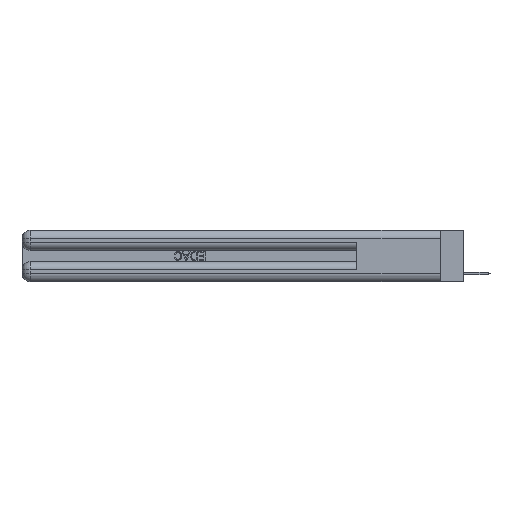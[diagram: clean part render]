
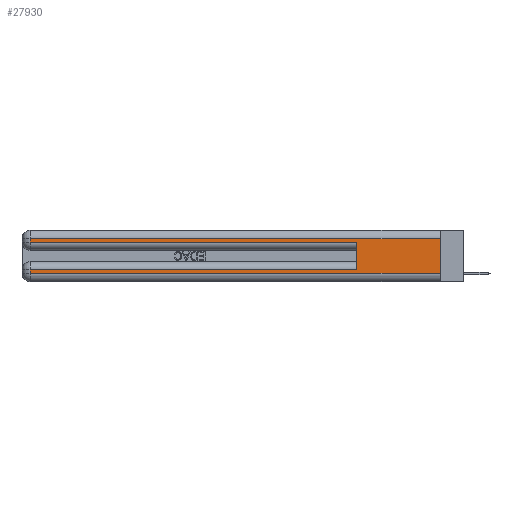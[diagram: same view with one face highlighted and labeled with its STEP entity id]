
A CAD part, left-side view. The second image highlights one B-rep face of the part: STEP entity #27930.
In plain terms, the highlighted planar face has unit normal (-1, 0, 0).
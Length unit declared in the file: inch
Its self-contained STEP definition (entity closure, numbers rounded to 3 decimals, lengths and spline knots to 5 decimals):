
#1215 = ORIENTED_EDGE ( 'NONE', *, *, #13368, .F. ) ;
#2618 = LINE ( 'NONE', #22978, #9329 ) ;
#2910 = CARTESIAN_POINT ( 'NONE',  ( 0., 2.94, 0.37 ) ) ;
#3831 = VECTOR ( 'NONE', #19390, 39.37008 ) ;
#4505 = DIRECTION ( 'NONE',  ( 0., 0., 1. ) ) ;
#5146 = CARTESIAN_POINT ( 'NONE',  ( 0., 2.94, 0.06 ) ) ;
#5337 = EDGE_CURVE ( 'NONE', #7466, #20631, #20648, .T. ) ;
#5552 = ORIENTED_EDGE ( 'NONE', *, *, #7578, .T. ) ;
#6166 = VERTEX_POINT ( 'NONE', #7833 ) ;
#6330 = FACE_OUTER_BOUND ( 'NONE', #6844, .T. ) ;
#6465 = CARTESIAN_POINT ( 'NONE',  ( 0., 0.6, 0.085 ) ) ;
#6713 = ORIENTED_EDGE ( 'NONE', *, *, #5337, .T. ) ;
#6844 = EDGE_LOOP ( 'NONE', ( #1215, #6713, #9039, #5552, #26929, #23325, #10239, #13207 ) ) ;
#7064 = DIRECTION ( 'NONE',  ( 0., 1., 0. ) ) ;
#7466 = VERTEX_POINT ( 'NONE', #10834 ) ;
#7518 = VECTOR ( 'NONE', #18152, 39.37008 ) ;
#7578 = EDGE_CURVE ( 'NONE', #30555, #27766, #29322, .T. ) ;
#7833 = CARTESIAN_POINT ( 'NONE',  ( 0., 2.94, 0.085 ) ) ;
#7868 = LINE ( 'NONE', #21384, #28889 ) ;
#7898 = CARTESIAN_POINT ( 'NONE',  ( 0., 2.94, 0.31 ) ) ;
#8642 = DIRECTION ( 'NONE',  ( 0., 1., 0. ) ) ;
#9039 = ORIENTED_EDGE ( 'NONE', *, *, #16519, .T. ) ;
#9329 = VECTOR ( 'NONE', #7064, 39.37008 ) ;
#9501 = CARTESIAN_POINT ( 'NONE',  ( 0., 2.94, 0.37 ) ) ;
#10239 = ORIENTED_EDGE ( 'NONE', *, *, #20258, .T. ) ;
#10388 = DIRECTION ( 'NONE',  ( 0., 0., -1. ) ) ;
#10834 = CARTESIAN_POINT ( 'NONE',  ( 0., 0., 0.31 ) ) ;
#11643 = DIRECTION ( 'NONE',  ( 0., 0., -1. ) ) ;
#12495 = VECTOR ( 'NONE', #18822, 39.37008 ) ;
#12959 = EDGE_CURVE ( 'NONE', #17915, #25589, #19751, .T. ) ;
#13207 = ORIENTED_EDGE ( 'NONE', *, *, #12959, .T. ) ;
#13304 = VECTOR ( 'NONE', #8642, 39.37008 ) ;
#13368 = EDGE_CURVE ( 'NONE', #7466, #25589, #7868, .T. ) ;
#13879 = VECTOR ( 'NONE', #11643, 39.37008 ) ;
#14038 = CARTESIAN_POINT ( 'NONE',  ( 0., 0.6, 0.285 ) ) ;
#14479 = EDGE_CURVE ( 'NONE', #26904, #6166, #2618, .T. ) ;
#15203 = LINE ( 'NONE', #16037, #24009 ) ;
#15687 = CARTESIAN_POINT ( 'NONE',  ( 0., 0., 0.06 ) ) ;
#15903 = CARTESIAN_POINT ( 'NONE',  ( 0., 2.94, 0.285 ) ) ;
#16037 = CARTESIAN_POINT ( 'NONE',  ( 0., 0.6, 0.145 ) ) ;
#16519 = EDGE_CURVE ( 'NONE', #20631, #30555, #24879, .T. ) ;
#16583 = DIRECTION ( 'NONE',  ( 0., 0., -1. ) ) ;
#17915 = VERTEX_POINT ( 'NONE', #5146 ) ;
#18152 = DIRECTION ( 'NONE',  ( 0., -1., 0. ) ) ;
#18822 = DIRECTION ( 'NONE',  ( 0., 0., -1. ) ) ;
#19390 = DIRECTION ( 'NONE',  ( 0., -1., 0. ) ) ;
#19583 = PLANE ( 'NONE',  #29483 ) ;
#19751 = LINE ( 'NONE', #15687, #7518 ) ;
#20258 = EDGE_CURVE ( 'NONE', #6166, #17915, #23531, .T. ) ;
#20631 = VERTEX_POINT ( 'NONE', #7898 ) ;
#20648 = LINE ( 'NONE', #25354, #13304 ) ;
#21384 = CARTESIAN_POINT ( 'NONE',  ( 0., 0., 0.37 ) ) ;
#22978 = CARTESIAN_POINT ( 'NONE',  ( 0., 0., 0.085 ) ) ;
#22984 = CARTESIAN_POINT ( 'NONE',  ( 0., 0., 0.06 ) ) ;
#23325 = ORIENTED_EDGE ( 'NONE', *, *, #14479, .T. ) ;
#23531 = LINE ( 'NONE', #9501, #12495 ) ;
#23765 = CARTESIAN_POINT ( 'NONE',  ( 0., 0., 0.285 ) ) ;
#24009 = VECTOR ( 'NONE', #4505, 39.37008 ) ;
#24574 = CARTESIAN_POINT ( 'NONE',  ( 0., 0., 0.37 ) ) ;
#24879 = LINE ( 'NONE', #2910, #13879 ) ;
#25354 = CARTESIAN_POINT ( 'NONE',  ( 0., 0., 0.31 ) ) ;
#25589 = VERTEX_POINT ( 'NONE', #22984 ) ;
#26904 = VERTEX_POINT ( 'NONE', #6465 ) ;
#26929 = ORIENTED_EDGE ( 'NONE', *, *, #29841, .F. ) ;
#27766 = VERTEX_POINT ( 'NONE', #14038 ) ;
#27930 = ADVANCED_FACE ( 'NONE', ( #6330 ), #19583, .F. ) ;
#28889 = VECTOR ( 'NONE', #16583, 39.37008 ) ;
#29298 = DIRECTION ( 'NONE',  ( 1., 0., 0. ) ) ;
#29322 = LINE ( 'NONE', #23765, #3831 ) ;
#29483 = AXIS2_PLACEMENT_3D ( 'NONE', #24574, #29298, #10388 ) ;
#29841 = EDGE_CURVE ( 'NONE', #26904, #27766, #15203, .T. ) ;
#30555 = VERTEX_POINT ( 'NONE', #15903 ) ;
